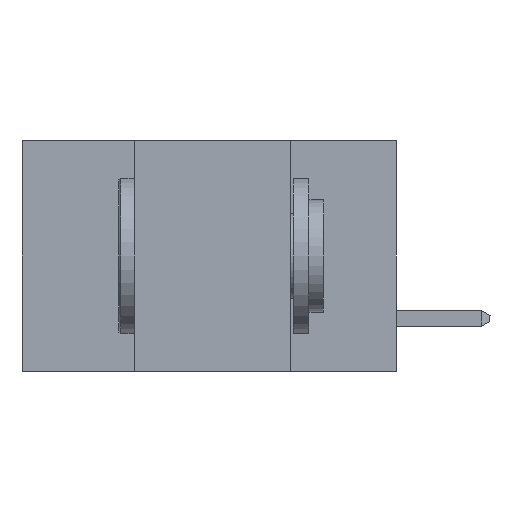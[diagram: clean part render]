
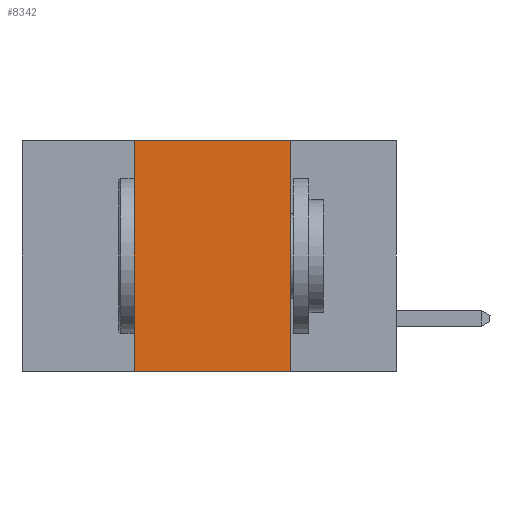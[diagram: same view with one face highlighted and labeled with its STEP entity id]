
A CAD part, left-side view. The second image highlights one B-rep face of the part: STEP entity #8342.
In plain terms, the highlighted planar face has unit normal (-1, 0, 0).
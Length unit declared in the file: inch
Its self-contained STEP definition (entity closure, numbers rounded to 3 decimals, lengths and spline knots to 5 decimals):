
#275 = LINE ( 'NONE', #909, #10915 ) ;
#366 = VERTEX_POINT ( 'NONE', #11661 ) ;
#909 = CARTESIAN_POINT ( 'NONE',  ( 0., 0.6, -0.37 ) ) ;
#937 = CARTESIAN_POINT ( 'NONE',  ( 0., 0.6, 0. ) ) ;
#966 = VERTEX_POINT ( 'NONE', #14193 ) ;
#1238 = AXIS2_PLACEMENT_3D ( 'NONE', #937, #2255, #11165 ) ;
#1679 = CARTESIAN_POINT ( 'NONE',  ( 0., 0.42, -0.37 ) ) ;
#2255 = DIRECTION ( 'NONE',  ( 1., 0., 0. ) ) ;
#2712 = VERTEX_POINT ( 'NONE', #5839 ) ;
#3006 = DIRECTION ( 'NONE',  ( 0., 0., 1. ) ) ;
#3472 = LINE ( 'NONE', #1679, #16317 ) ;
#4548 = LINE ( 'NONE', #12450, #7494 ) ;
#5164 = ORIENTED_EDGE ( 'NONE', *, *, #15635, .F. ) ;
#5326 = EDGE_CURVE ( 'NONE', #5723, #366, #9192, .T. ) ;
#5723 = VERTEX_POINT ( 'NONE', #7656 ) ;
#5820 = FACE_OUTER_BOUND ( 'NONE', #9840, .T. ) ;
#5839 = CARTESIAN_POINT ( 'NONE',  ( 0., 0.17, -0.37 ) ) ;
#5847 = ORIENTED_EDGE ( 'NONE', *, *, #5326, .F. ) ;
#6270 = ORIENTED_EDGE ( 'NONE', *, *, #10420, .T. ) ;
#7277 = ORIENTED_EDGE ( 'NONE', *, *, #8728, .F. ) ;
#7494 = VECTOR ( 'NONE', #14884, 39.37008 ) ;
#7656 = CARTESIAN_POINT ( 'NONE',  ( 0., 0.42, 0. ) ) ;
#8342 = ADVANCED_FACE ( 'NONE', ( #5820 ), #12299, .F. ) ;
#8728 = EDGE_CURVE ( 'NONE', #966, #5723, #3472, .T. ) ;
#9192 = LINE ( 'NONE', #10333, #15356 ) ;
#9840 = EDGE_LOOP ( 'NONE', ( #5164, #5847, #7277, #6270 ) ) ;
#10333 = CARTESIAN_POINT ( 'NONE',  ( 0., 0.6, 0. ) ) ;
#10420 = EDGE_CURVE ( 'NONE', #966, #2712, #275, .T. ) ;
#10915 = VECTOR ( 'NONE', #12318, 39.37008 ) ;
#11165 = DIRECTION ( 'NONE',  ( 0., 0., -1. ) ) ;
#11661 = CARTESIAN_POINT ( 'NONE',  ( 0., 0.17, 0. ) ) ;
#12299 = PLANE ( 'NONE',  #1238 ) ;
#12318 = DIRECTION ( 'NONE',  ( 0., -1., 0. ) ) ;
#12450 = CARTESIAN_POINT ( 'NONE',  ( 0., 0.17, -0.37 ) ) ;
#14053 = DIRECTION ( 'NONE',  ( 0., -1., 0. ) ) ;
#14193 = CARTESIAN_POINT ( 'NONE',  ( 0., 0.42, -0.37 ) ) ;
#14884 = DIRECTION ( 'NONE',  ( 0., 0., -1. ) ) ;
#15356 = VECTOR ( 'NONE', #14053, 39.37008 ) ;
#15635 = EDGE_CURVE ( 'NONE', #366, #2712, #4548, .T. ) ;
#16317 = VECTOR ( 'NONE', #3006, 39.37008 ) ;
